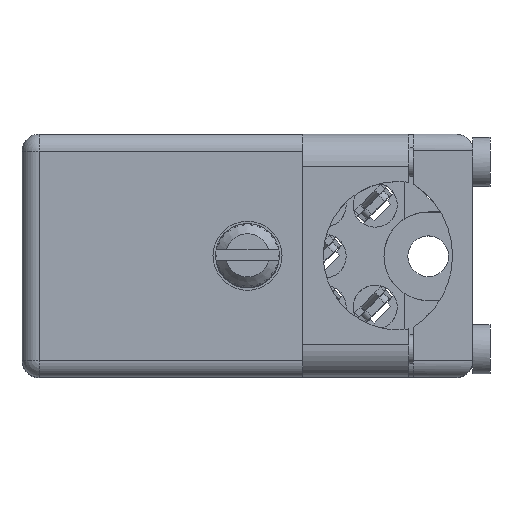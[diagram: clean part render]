
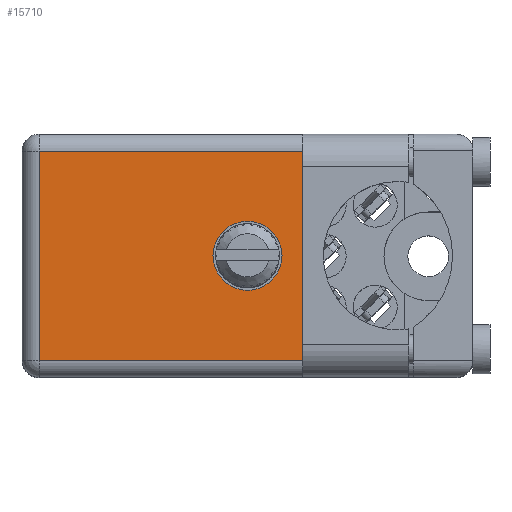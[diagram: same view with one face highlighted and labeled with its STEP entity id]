
A CAD part, top view. The second image highlights one B-rep face of the part: STEP entity #15710.
In plain terms, the highlighted face is planar.
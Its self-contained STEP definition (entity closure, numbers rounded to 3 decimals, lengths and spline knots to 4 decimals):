
#2465 = VECTOR ( 'NONE', #69580, 39.3701 ) ;
#4179 = EDGE_CURVE ( 'NONE', #124770, #65062, #43265, .T. ) ;
#4289 = VERTEX_POINT ( 'NONE', #20665 ) ;
#5827 = EDGE_CURVE ( 'NONE', #19324, #159563, #139519, .T. ) ;
#12980 = CARTESIAN_POINT ( 'NONE',  ( 0.865, 0.906, -0.1125 ) ) ;
#13313 = LINE ( 'NONE', #98685, #70608 ) ;
#13329 = VERTEX_POINT ( 'NONE', #78503 ) ;
#14624 = CARTESIAN_POINT ( 'NONE',  ( 0.865, 0.906, -0.1125 ) ) ;
#15710 = ADVANCED_FACE ( 'NONE', ( #114947, #57706 ), #112182, .T. ) ;
#16074 = ORIENTED_EDGE ( 'NONE', *, *, #5827, .T. ) ;
#18934 = CARTESIAN_POINT ( 'NONE',  ( 0.6625, 0.906, -0.459 ) ) ;
#19324 = VERTEX_POINT ( 'NONE', #115063 ) ;
#20388 = VERTEX_POINT ( 'NONE', #120571 ) ;
#20665 = CARTESIAN_POINT ( 'NONE',  ( 0.865, 0.906, -0.6025 ) ) ;
#20903 = EDGE_CURVE ( 'NONE', #19324, #155919, #13313, .T. ) ;
#23278 = LINE ( 'NONE', #53286, #46601 ) ;
#27869 = ORIENTED_EDGE ( 'NONE', *, *, #20903, .F. ) ;
#27937 = DIRECTION ( 'NONE',  ( 0., 0., -1. ) ) ;
#30468 = AXIS2_PLACEMENT_3D ( 'NONE', #169412, #31376, #144959 ) ;
#31376 = DIRECTION ( 'NONE',  ( 0., 1., 0. ) ) ;
#36576 = EDGE_CURVE ( 'NONE', #159563, #4289, #156508, .T. ) ;
#37236 = DIRECTION ( 'NONE',  ( 0., 0., 1. ) ) ;
#37900 = AXIS2_PLACEMENT_3D ( 'NONE', #109469, #165784, #37236 ) ;
#39322 = CARTESIAN_POINT ( 'NONE',  ( 1.15, 0.906, -0.665 ) ) ;
#43265 = LINE ( 'NONE', #169976, #2465 ) ;
#46601 = VECTOR ( 'NONE', #180883, 39.3701 ) ;
#47160 = CARTESIAN_POINT ( 'NONE',  ( 1.15, 0.906, -0.05 ) ) ;
#48012 = CARTESIAN_POINT ( 'NONE',  ( 1.15, 0.906, -0.05 ) ) ;
#53286 = CARTESIAN_POINT ( 'NONE',  ( 0., 0.906, -0.665 ) ) ;
#55017 = DIRECTION ( 'NONE',  ( -1., 0., 0. ) ) ;
#55138 = CARTESIAN_POINT ( 'NONE',  ( 0.05, 0.906, -0.715 ) ) ;
#57706 = FACE_BOUND ( 'NONE', #137138, .T. ) ;
#58931 = ORIENTED_EDGE ( 'NONE', *, *, #168046, .T. ) ;
#65062 = VERTEX_POINT ( 'NONE', #101098 ) ;
#69580 = DIRECTION ( 'NONE',  ( 0., 0., 1. ) ) ;
#70608 = VECTOR ( 'NONE', #125910, 39.3701 ) ;
#74622 = VECTOR ( 'NONE', #179778, 39.3701 ) ;
#76669 = LINE ( 'NONE', #164802, #74622 ) ;
#78503 = CARTESIAN_POINT ( 'NONE',  ( 0.05, 0.906, -0.665 ) ) ;
#79998 = CIRCLE ( 'NONE', #37900, 0.1015 ) ;
#86536 = CIRCLE ( 'NONE', #89504, 0.1015 ) ;
#89386 = EDGE_CURVE ( 'NONE', #177049, #130900, #79998, .T. ) ;
#89504 = AXIS2_PLACEMENT_3D ( 'NONE', #145614, #185063, #99720 ) ;
#93346 = ORIENTED_EDGE ( 'NONE', *, *, #150499, .T. ) ;
#94424 = CARTESIAN_POINT ( 'NONE',  ( 0.865, 0.906, -0.1125 ) ) ;
#98685 = CARTESIAN_POINT ( 'NONE',  ( 1.15, 0.906, -0.715 ) ) ;
#99720 = DIRECTION ( 'NONE',  ( 0., 0., 1. ) ) ;
#100613 = VECTOR ( 'NONE', #171447, 39.3701 ) ;
#101098 = CARTESIAN_POINT ( 'NONE',  ( 1.15, 0.906, -0.6025 ) ) ;
#107415 = ORIENTED_EDGE ( 'NONE', *, *, #4179, .F. ) ;
#109331 = ORIENTED_EDGE ( 'NONE', *, *, #126411, .T. ) ;
#109469 = CARTESIAN_POINT ( 'NONE',  ( 0.6625, 0.906, -0.3575 ) ) ;
#110605 = ORIENTED_EDGE ( 'NONE', *, *, #166342, .F. ) ;
#112182 = PLANE ( 'NONE',  #30468 ) ;
#113810 = ORIENTED_EDGE ( 'NONE', *, *, #36576, .T. ) ;
#114831 = EDGE_LOOP ( 'NONE', ( #93346, #172340, #27869, #16074, #113810, #58931, #107415, #109331 ) ) ;
#114947 = FACE_OUTER_BOUND ( 'NONE', #114831, .T. ) ;
#115063 = CARTESIAN_POINT ( 'NONE',  ( 1.15, 0.906, -0.1125 ) ) ;
#118462 = LINE ( 'NONE', #47160, #173697 ) ;
#120571 = CARTESIAN_POINT ( 'NONE',  ( 0.05, 0.906, -0.05 ) ) ;
#124770 = VERTEX_POINT ( 'NONE', #39322 ) ;
#125910 = DIRECTION ( 'NONE',  ( 0., 0., 1. ) ) ;
#126411 = EDGE_CURVE ( 'NONE', #124770, #13329, #23278, .T. ) ;
#130900 = VERTEX_POINT ( 'NONE', #18934 ) ;
#133492 = DIRECTION ( 'NONE',  ( 1., 0., 0. ) ) ;
#134009 = VECTOR ( 'NONE', #55017, 39.3701 ) ;
#137138 = EDGE_LOOP ( 'NONE', ( #182250, #110605 ) ) ;
#139519 = LINE ( 'NONE', #14624, #134009 ) ;
#144959 = DIRECTION ( 'NONE',  ( 0., 0., 1. ) ) ;
#145614 = CARTESIAN_POINT ( 'NONE',  ( 0.6625, 0.906, -0.3575 ) ) ;
#150499 = EDGE_CURVE ( 'NONE', #13329, #20388, #168677, .T. ) ;
#152628 = CARTESIAN_POINT ( 'NONE',  ( 0.6625, 0.906, -0.256 ) ) ;
#155919 = VERTEX_POINT ( 'NONE', #48012 ) ;
#156508 = LINE ( 'NONE', #12980, #180277 ) ;
#159563 = VERTEX_POINT ( 'NONE', #94424 ) ;
#164802 = CARTESIAN_POINT ( 'NONE',  ( 0.865, 0.906, -0.6025 ) ) ;
#165784 = DIRECTION ( 'NONE',  ( 0., 1., 0. ) ) ;
#166342 = EDGE_CURVE ( 'NONE', #130900, #177049, #86536, .T. ) ;
#168046 = EDGE_CURVE ( 'NONE', #4289, #65062, #76669, .T. ) ;
#168677 = LINE ( 'NONE', #55138, #100613 ) ;
#169412 = CARTESIAN_POINT ( 'NONE',  ( 0., 0.906, -0.715 ) ) ;
#169976 = CARTESIAN_POINT ( 'NONE',  ( 1.15, 0.906, -0.715 ) ) ;
#171447 = DIRECTION ( 'NONE',  ( 0., 0., 1. ) ) ;
#171776 = EDGE_CURVE ( 'NONE', #20388, #155919, #118462, .T. ) ;
#172340 = ORIENTED_EDGE ( 'NONE', *, *, #171776, .T. ) ;
#173697 = VECTOR ( 'NONE', #133492, 39.3701 ) ;
#177049 = VERTEX_POINT ( 'NONE', #152628 ) ;
#179778 = DIRECTION ( 'NONE',  ( 1., 0., 0. ) ) ;
#180277 = VECTOR ( 'NONE', #27937, 39.3701 ) ;
#180883 = DIRECTION ( 'NONE',  ( -1., 0., 0. ) ) ;
#182250 = ORIENTED_EDGE ( 'NONE', *, *, #89386, .F. ) ;
#185063 = DIRECTION ( 'NONE',  ( 0., 1., 0. ) ) ;
